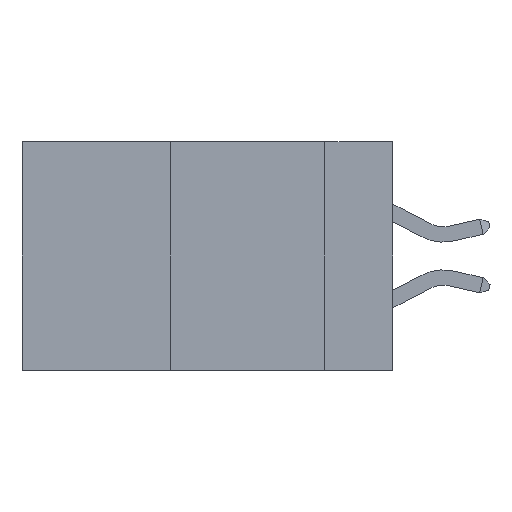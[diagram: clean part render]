
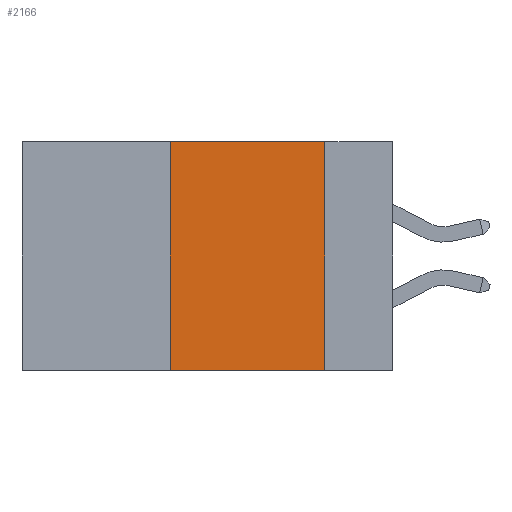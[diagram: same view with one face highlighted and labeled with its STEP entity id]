
A CAD part, left-side view. The second image highlights one B-rep face of the part: STEP entity #2166.
In plain terms, the highlighted planar face has unit normal (-1, 0, 0).
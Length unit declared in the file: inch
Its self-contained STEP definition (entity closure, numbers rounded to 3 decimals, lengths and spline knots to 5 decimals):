
#102 = VERTEX_POINT ( 'NONE', #17024 ) ;
#704 = DIRECTION ( 'NONE',  ( 1., 0., 0. ) ) ;
#2166 = ADVANCED_FACE ( 'NONE', ( #15504 ), #4961, .F. ) ;
#2428 = DIRECTION ( 'NONE',  ( 0., -1., 0. ) ) ;
#3473 = CARTESIAN_POINT ( 'NONE',  ( 0., 0.6, 0. ) ) ;
#3930 = CARTESIAN_POINT ( 'NONE',  ( 0., 0.6, -0.37 ) ) ;
#3934 = EDGE_LOOP ( 'NONE', ( #10286, #7237, #16230, #12343 ) ) ;
#4497 = EDGE_CURVE ( 'NONE', #15437, #12584, #14422, .T. ) ;
#4961 = PLANE ( 'NONE',  #11205 ) ;
#5016 = LINE ( 'NONE', #11186, #12740 ) ;
#7237 = ORIENTED_EDGE ( 'NONE', *, *, #4497, .F. ) ;
#9315 = LINE ( 'NONE', #9996, #17387 ) ;
#9485 = CARTESIAN_POINT ( 'NONE',  ( 0., 0.11, -0.37 ) ) ;
#9996 = CARTESIAN_POINT ( 'NONE',  ( 0., 0.36, 0. ) ) ;
#10286 = ORIENTED_EDGE ( 'NONE', *, *, #20077, .F. ) ;
#10871 = VERTEX_POINT ( 'NONE', #9485 ) ;
#10997 = LINE ( 'NONE', #3930, #14803 ) ;
#11186 = CARTESIAN_POINT ( 'NONE',  ( 0., 0.11, 0. ) ) ;
#11205 = AXIS2_PLACEMENT_3D ( 'NONE', #3473, #704, #17632 ) ;
#11651 = DIRECTION ( 'NONE',  ( 0., 0., 1. ) ) ;
#11704 = EDGE_CURVE ( 'NONE', #102, #15437, #9315, .T. ) ;
#11934 = DIRECTION ( 'NONE',  ( 0., -1., 0. ) ) ;
#12343 = ORIENTED_EDGE ( 'NONE', *, *, #18001, .T. ) ;
#12584 = VERTEX_POINT ( 'NONE', #18718 ) ;
#12649 = CARTESIAN_POINT ( 'NONE',  ( 0., 0.36, 0. ) ) ;
#12740 = VECTOR ( 'NONE', #12849, 39.37008 ) ;
#12849 = DIRECTION ( 'NONE',  ( 0., 0., -1. ) ) ;
#14422 = LINE ( 'NONE', #19837, #14915 ) ;
#14803 = VECTOR ( 'NONE', #2428, 39.37008 ) ;
#14915 = VECTOR ( 'NONE', #11934, 39.37008 ) ;
#15437 = VERTEX_POINT ( 'NONE', #12649 ) ;
#15504 = FACE_OUTER_BOUND ( 'NONE', #3934, .T. ) ;
#16230 = ORIENTED_EDGE ( 'NONE', *, *, #11704, .F. ) ;
#17024 = CARTESIAN_POINT ( 'NONE',  ( 0., 0.36, -0.37 ) ) ;
#17387 = VECTOR ( 'NONE', #11651, 39.37008 ) ;
#17632 = DIRECTION ( 'NONE',  ( 0., 0., -1. ) ) ;
#18001 = EDGE_CURVE ( 'NONE', #102, #10871, #10997, .T. ) ;
#18718 = CARTESIAN_POINT ( 'NONE',  ( 0., 0.11, 0. ) ) ;
#19837 = CARTESIAN_POINT ( 'NONE',  ( 0., 0.6, 0. ) ) ;
#20077 = EDGE_CURVE ( 'NONE', #12584, #10871, #5016, .T. ) ;
